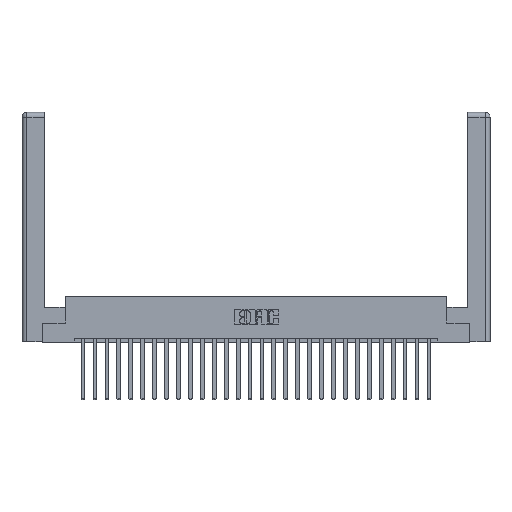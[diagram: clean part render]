
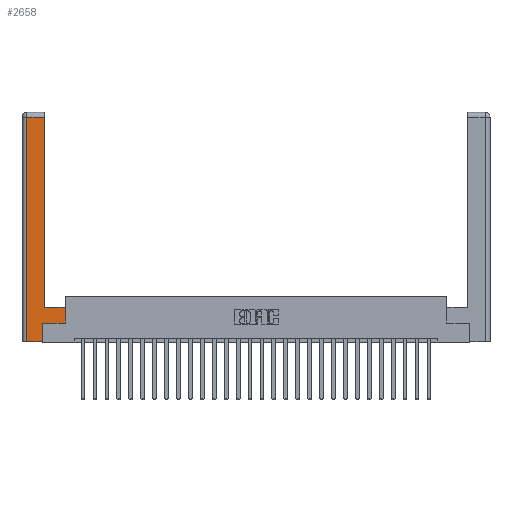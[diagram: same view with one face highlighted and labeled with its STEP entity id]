
A CAD part, top view. The second image highlights one B-rep face of the part: STEP entity #2658.
In plain terms, the highlighted planar face has unit normal (0, 0, 1).
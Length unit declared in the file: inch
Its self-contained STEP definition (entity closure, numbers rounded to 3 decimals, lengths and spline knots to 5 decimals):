
#129 = ORIENTED_EDGE ( 'NONE', *, *, #21629, .T. ) ;
#357 = VERTEX_POINT ( 'NONE', #15725 ) ;
#645 = CARTESIAN_POINT ( 'NONE',  ( 0.565, 0.245, 0. ) ) ;
#696 = DIRECTION ( 'NONE',  ( -1., 0., 0. ) ) ;
#1159 = VECTOR ( 'NONE', #15146, 39.37008 ) ;
#1277 = ORIENTED_EDGE ( 'NONE', *, *, #26592, .T. ) ;
#1466 = ORIENTED_EDGE ( 'NONE', *, *, #15171, .T. ) ;
#1591 = LINE ( 'NONE', #645, #26938 ) ;
#2638 = DIRECTION ( 'NONE',  ( 0., 1., 0. ) ) ;
#2658 = ADVANCED_FACE ( 'NONE', ( #7751 ), #23805, .F. ) ;
#2846 = DIRECTION ( 'NONE',  ( 0., 0., -1. ) ) ;
#3236 = AXIS2_PLACEMENT_3D ( 'NONE', #17360, #2846, #696 ) ;
#3628 = VECTOR ( 'NONE', #5361, 39.37008 ) ;
#4313 = CARTESIAN_POINT ( 'NONE',  ( 0.0615, 0., 0. ) ) ;
#4857 = VERTEX_POINT ( 'NONE', #22984 ) ;
#5361 = DIRECTION ( 'NONE',  ( 0., 1., 0. ) ) ;
#6135 = VERTEX_POINT ( 'NONE', #16718 ) ;
#6487 = LINE ( 'NONE', #25725, #26888 ) ;
#6641 = DIRECTION ( 'NONE',  ( -1., 0., 0. ) ) ;
#7568 = CARTESIAN_POINT ( 'NONE',  ( 0.565, 0.45, 0. ) ) ;
#7751 = FACE_OUTER_BOUND ( 'NONE', #9302, .T. ) ;
#8887 = VERTEX_POINT ( 'NONE', #24482 ) ;
#8907 = LINE ( 'NONE', #7568, #3628 ) ;
#9166 = DIRECTION ( 'NONE',  ( 1., 0., 0. ) ) ;
#9252 = LINE ( 'NONE', #24799, #24029 ) ;
#9302 = EDGE_LOOP ( 'NONE', ( #11961, #24990, #10606, #1277, #1466, #25088, #129, #15625 ) ) ;
#9751 = VECTOR ( 'NONE', #6641, 39.37008 ) ;
#10103 = CARTESIAN_POINT ( 'NONE',  ( 0.0615, 2.94, 0. ) ) ;
#10117 = CARTESIAN_POINT ( 'NONE',  ( 0.565, 0.45, 0. ) ) ;
#10358 = DIRECTION ( 'NONE',  ( -1., 0., 0. ) ) ;
#10606 = ORIENTED_EDGE ( 'NONE', *, *, #16449, .T. ) ;
#11288 = CARTESIAN_POINT ( 'NONE',  ( 0.265, 0.245, 0. ) ) ;
#11961 = ORIENTED_EDGE ( 'NONE', *, *, #13386, .T. ) ;
#12024 = VERTEX_POINT ( 'NONE', #12586 ) ;
#12378 = DIRECTION ( 'NONE',  ( 0., 1., 0. ) ) ;
#12586 = CARTESIAN_POINT ( 'NONE',  ( 0.295, 2.94, 0. ) ) ;
#12928 = CARTESIAN_POINT ( 'NONE',  ( 0.265, 0.245, 0. ) ) ;
#13386 = EDGE_CURVE ( 'NONE', #4857, #12024, #9252, .T. ) ;
#14137 = DIRECTION ( 'NONE',  ( 1., 0., 0. ) ) ;
#15146 = DIRECTION ( 'NONE',  ( 0., -1., 0. ) ) ;
#15171 = EDGE_CURVE ( 'NONE', #16318, #15227, #26214, .T. ) ;
#15227 = VERTEX_POINT ( 'NONE', #11288 ) ;
#15625 = ORIENTED_EDGE ( 'NONE', *, *, #17228, .T. ) ;
#15725 = CARTESIAN_POINT ( 'NONE',  ( 0.0615, 0., 0. ) ) ;
#15976 = VECTOR ( 'NONE', #10358, 39.37008 ) ;
#16318 = VERTEX_POINT ( 'NONE', #22787 ) ;
#16449 = EDGE_CURVE ( 'NONE', #6135, #357, #24537, .T. ) ;
#16718 = CARTESIAN_POINT ( 'NONE',  ( 0.0615, 2.94, 0. ) ) ;
#17228 = EDGE_CURVE ( 'NONE', #23641, #4857, #25159, .T. ) ;
#17360 = CARTESIAN_POINT ( 'NONE',  ( 0., 0., 0. ) ) ;
#18849 = EDGE_CURVE ( 'NONE', #12024, #6135, #22208, .T. ) ;
#18974 = VECTOR ( 'NONE', #2638, 39.37008 ) ;
#21629 = EDGE_CURVE ( 'NONE', #8887, #23641, #8907, .T. ) ;
#22199 = EDGE_CURVE ( 'NONE', #15227, #8887, #1591, .T. ) ;
#22208 = LINE ( 'NONE', #10103, #15976 ) ;
#22787 = CARTESIAN_POINT ( 'NONE',  ( 0.265, 0., 0. ) ) ;
#22984 = CARTESIAN_POINT ( 'NONE',  ( 0.295, 0.45, 0. ) ) ;
#23641 = VERTEX_POINT ( 'NONE', #10117 ) ;
#23642 = CARTESIAN_POINT ( 'NONE',  ( 0.295, 0.45, 0. ) ) ;
#23805 = PLANE ( 'NONE',  #3236 ) ;
#24029 = VECTOR ( 'NONE', #12378, 39.37008 ) ;
#24482 = CARTESIAN_POINT ( 'NONE',  ( 0.565, 0.245, 0. ) ) ;
#24537 = LINE ( 'NONE', #4313, #1159 ) ;
#24799 = CARTESIAN_POINT ( 'NONE',  ( 0.295, 3., 0. ) ) ;
#24990 = ORIENTED_EDGE ( 'NONE', *, *, #18849, .T. ) ;
#25088 = ORIENTED_EDGE ( 'NONE', *, *, #22199, .T. ) ;
#25159 = LINE ( 'NONE', #23642, #9751 ) ;
#25725 = CARTESIAN_POINT ( 'NONE',  ( 0.265, 0., 0. ) ) ;
#26214 = LINE ( 'NONE', #12928, #18974 ) ;
#26592 = EDGE_CURVE ( 'NONE', #357, #16318, #6487, .T. ) ;
#26888 = VECTOR ( 'NONE', #14137, 39.37008 ) ;
#26938 = VECTOR ( 'NONE', #9166, 39.37008 ) ;
